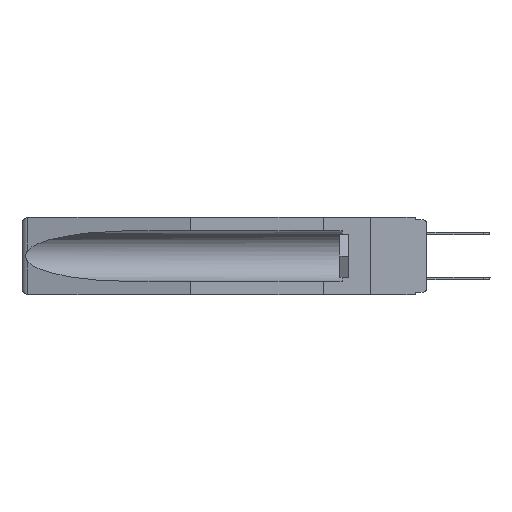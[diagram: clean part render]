
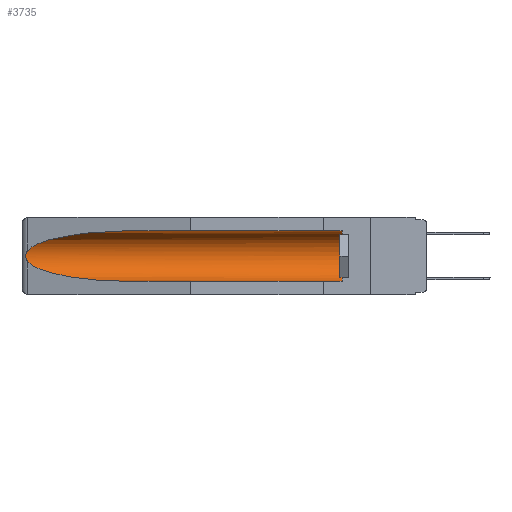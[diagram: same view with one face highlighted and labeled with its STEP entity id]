
A CAD part, left-side view. The second image highlights one B-rep face of the part: STEP entity #3735.
In plain terms, the highlighted cylindrical face has radius 2.857 mm (diameter 5.715 mm), a partial arc.
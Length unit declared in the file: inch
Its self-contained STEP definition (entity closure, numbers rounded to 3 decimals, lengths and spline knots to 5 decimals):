
#215 = CARTESIAN_POINT ( 'NONE',  ( 0.155, -0.30754, -0.1715 ) ) ;
#301 = ORIENTED_EDGE ( 'NONE', *, *, #2687, .T. ) ;
#507 = CARTESIAN_POINT ( 'NONE',  ( 0.155, 1.07973, -0.059 ) ) ;
#769 = CARTESIAN_POINT ( 'NONE',  ( 0.26537, 1.52718, -0.19328 ) ) ;
#1068 = EDGE_CURVE ( 'NONE', #3208, #7770, #7361, .T. ) ;
#1310 = CARTESIAN_POINT ( 'NONE',  ( 0.155, 0.126, -0.059 ) ) ;
#2113 = CARTESIAN_POINT ( 'NONE',  ( 0.25451, 1.48313, -0.09465 ) ) ;
#2233 = CARTESIAN_POINT ( 'NONE',  ( 0.155, 1.07973, -0.059 ) ) ;
#2687 = EDGE_CURVE ( 'NONE', #13843, #2770, #3373, .T. ) ;
#2770 = VERTEX_POINT ( 'NONE', #13137 ) ;
#3208 = VERTEX_POINT ( 'NONE', #8266 ) ;
#3314 = CARTESIAN_POINT ( 'NONE',  ( 0.2673, 1.53269, -0.17917 ) ) ;
#3373 =( BOUNDED_CURVE ( )  B_SPLINE_CURVE ( 3, ( #507, #10015, #2113, #11333 ),
 .UNSPECIFIED., .F., .F. ) 
 B_SPLINE_CURVE_WITH_KNOTS ( ( 4, 4 ),
 ( 4.71239, 6.08839 ),
 .UNSPECIFIED. ) 
 CURVE ( )  GEOMETRIC_REPRESENTATION_ITEM ( )  RATIONAL_B_SPLINE_CURVE ( ( 1., 0.848, 0.848, 1. ) ) 
 REPRESENTATION_ITEM ( '' )  );
#3553 = DIRECTION ( 'NONE',  ( 0., -1., 0. ) ) ;
#3735 = ADVANCED_FACE ( 'NONE', ( #11941 ), #13955, .F. ) ;
#3796 = CARTESIAN_POINT ( 'NONE',  ( 0.155, -0.30754, -0.284 ) ) ;
#5076 = EDGE_CURVE ( 'NONE', #7770, #13843, #5670, .T. ) ;
#5271 = VERTEX_POINT ( 'NONE', #9731 ) ;
#5306 = EDGE_LOOP ( 'NONE', ( #301, #18689, #19373, #19575, #13743, #17678 ) ) ;
#5651 = LINE ( 'NONE', #3796, #13856 ) ;
#5670 = LINE ( 'NONE', #11923, #15148 ) ;
#6213 = VERTEX_POINT ( 'NONE', #15991 ) ;
#6534 = DIRECTION ( 'NONE',  ( 0., 1., 0. ) ) ;
#6576 = CARTESIAN_POINT ( 'NONE',  ( 0.26537, 1.52718, -0.19328 ) ) ;
#7361 = CIRCLE ( 'NONE', #15230, 0.1125 ) ;
#7575 = CARTESIAN_POINT ( 'NONE',  ( 0.26597, 1.52961, -0.15275 ) ) ;
#7770 = VERTEX_POINT ( 'NONE', #1310 ) ;
#8266 = CARTESIAN_POINT ( 'NONE',  ( 0.155, 0.126, -0.284 ) ) ;
#8532 = CARTESIAN_POINT ( 'NONE',  ( 0.155, 0.126, -0.1715 ) ) ;
#9213 = AXIS2_PLACEMENT_3D ( 'NONE', #215, #6534, #16073 ) ;
#9731 = CARTESIAN_POINT ( 'NONE',  ( 0.155, 1.07973, -0.284 ) ) ;
#10015 = CARTESIAN_POINT ( 'NONE',  ( 0.21114, 1.30732, -0.059 ) ) ;
#10765 = CARTESIAN_POINT ( 'NONE',  ( 0.2673, 1.5327, -0.16383 ) ) ;
#11081 = EDGE_CURVE ( 'NONE', #2770, #6213, #13568, .T. ) ;
#11139 =( BOUNDED_CURVE ( )  B_SPLINE_CURVE ( 3, ( #769, #11925, #11785, #16828 ),
 .UNSPECIFIED., .F., .F. ) 
 B_SPLINE_CURVE_WITH_KNOTS ( ( 4, 4 ),
 ( 0.1948, 1.5708 ),
 .UNSPECIFIED. ) 
 CURVE ( )  GEOMETRIC_REPRESENTATION_ITEM ( )  RATIONAL_B_SPLINE_CURVE ( ( 1., 0.848, 0.848, 1. ) ) 
 REPRESENTATION_ITEM ( '' )  );
#11300 = CARTESIAN_POINT ( 'NONE',  ( 0.26597, 1.5296, -0.19026 ) ) ;
#11333 = CARTESIAN_POINT ( 'NONE',  ( 0.26537, 1.52718, -0.14972 ) ) ;
#11354 = EDGE_CURVE ( 'NONE', #3208, #5271, #5651, .T. ) ;
#11785 = CARTESIAN_POINT ( 'NONE',  ( 0.21114, 1.30732, -0.284 ) ) ;
#11923 = CARTESIAN_POINT ( 'NONE',  ( 0.155, -0.30754, -0.059 ) ) ;
#11925 = CARTESIAN_POINT ( 'NONE',  ( 0.25451, 1.48313, -0.24835 ) ) ;
#11941 = FACE_OUTER_BOUND ( 'NONE', #5306, .T. ) ;
#11971 = EDGE_CURVE ( 'NONE', #6213, #5271, #11139, .T. ) ;
#11974 = DIRECTION ( 'NONE',  ( 0., 1., 0. ) ) ;
#12405 = CARTESIAN_POINT ( 'NONE',  ( 0.26654, 1.53092, -0.15636 ) ) ;
#13137 = CARTESIAN_POINT ( 'NONE',  ( 0.26537, 1.52718, -0.14972 ) ) ;
#13568 = B_SPLINE_CURVE_WITH_KNOTS ( 'NONE', 3,
 ( #17114, #7575, #12405, #10765, #18795, #15709, #3314, #17458, #11300, #6576 ),
 .UNSPECIFIED., .F., .F.,
 ( 4, 2, 2, 2, 4 ),
 ( 0., 0.00029, 0.00058, 0.00087, 0.00117 ),
 .UNSPECIFIED. ) ;
#13743 = ORIENTED_EDGE ( 'NONE', *, *, #1068, .T. ) ;
#13843 = VERTEX_POINT ( 'NONE', #2233 ) ;
#13856 = VECTOR ( 'NONE', #11974, 39.37008 ) ;
#13955 = CYLINDRICAL_SURFACE ( 'NONE', #9213, 0.1125 ) ;
#14680 = DIRECTION ( 'NONE',  ( 0., 0., 1. ) ) ;
#15148 = VECTOR ( 'NONE', #19625, 39.37008 ) ;
#15230 = AXIS2_PLACEMENT_3D ( 'NONE', #8532, #3553, #14680 ) ;
#15709 = CARTESIAN_POINT ( 'NONE',  ( 0.2675, 1.53308, -0.17534 ) ) ;
#15991 = CARTESIAN_POINT ( 'NONE',  ( 0.26537, 1.52718, -0.19328 ) ) ;
#16073 = DIRECTION ( 'NONE',  ( 0., 0., 1. ) ) ;
#16828 = CARTESIAN_POINT ( 'NONE',  ( 0.155, 1.07973, -0.284 ) ) ;
#17114 = CARTESIAN_POINT ( 'NONE',  ( 0.26537, 1.52718, -0.14972 ) ) ;
#17458 = CARTESIAN_POINT ( 'NONE',  ( 0.26655, 1.53094, -0.18657 ) ) ;
#17678 = ORIENTED_EDGE ( 'NONE', *, *, #5076, .T. ) ;
#18689 = ORIENTED_EDGE ( 'NONE', *, *, #11081, .T. ) ;
#18795 = CARTESIAN_POINT ( 'NONE',  ( 0.2675, 1.53308, -0.16763 ) ) ;
#19373 = ORIENTED_EDGE ( 'NONE', *, *, #11971, .T. ) ;
#19575 = ORIENTED_EDGE ( 'NONE', *, *, #11354, .F. ) ;
#19625 = DIRECTION ( 'NONE',  ( 0., 1., 0. ) ) ;
